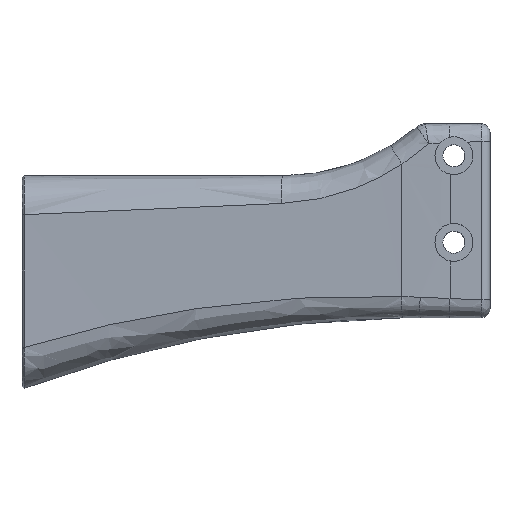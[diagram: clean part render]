
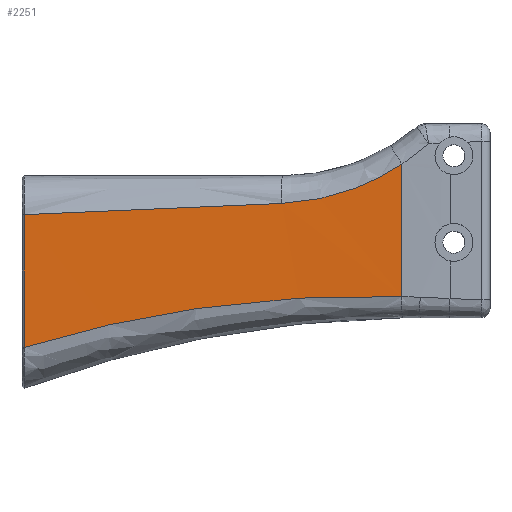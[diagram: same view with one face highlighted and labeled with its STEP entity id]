
A CAD part, left-side view. The second image highlights one B-rep face of the part: STEP entity #2251.
In plain terms, the highlighted cylindrical face has radius 3182.51 mm (diameter 6365.01 mm), a partial arc.
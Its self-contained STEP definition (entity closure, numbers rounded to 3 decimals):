
#116=B_SPLINE_CURVE_WITH_KNOTS('',3,(#3561,#3562,#3563,#3564),
 .UNSPECIFIED.,.F.,.F.,(4,4),(-1.419,-1.417),
 .UNSPECIFIED.);
#125=B_SPLINE_CURVE_WITH_KNOTS('',3,(#3805,#3806,#3807,#3808),
 .UNSPECIFIED.,.F.,.F.,(4,4),(0.05,6.025),
 .UNSPECIFIED.);
#128=B_SPLINE_CURVE_WITH_KNOTS('',3,(#3823,#3824,#3825,#3826,#3827),
 .UNSPECIFIED.,.F.,.F.,(4,1,4),(2.018,7.279,10.884),
 .UNSPECIFIED.);
#129=B_SPLINE_CURVE_WITH_KNOTS('',3,(#3830,#3831,#3832,#3833,#3834),
 .UNSPECIFIED.,.F.,.F.,(4,1,4),(6.025,7.294,8.985),
 .UNSPECIFIED.);
#303=FACE_OUTER_BOUND('',#443,.T.);
#443=EDGE_LOOP('',(#1794,#1795,#1796,#1797,#1798,#1799));
#614=LINE('',#3489,#779);
#631=LINE('',#3829,#796);
#779=VECTOR('',#2795,10.);
#796=VECTOR('',#2820,10.);
#1044=VERTEX_POINT('',#3486);
#1045=VERTEX_POINT('',#3488);
#1047=VERTEX_POINT('',#3537);
#1058=VERTEX_POINT('',#3804);
#1060=VERTEX_POINT('',#3822);
#1061=VERTEX_POINT('',#3828);
#1301=EDGE_CURVE('',#1044,#1045,#614,.T.);
#1307=EDGE_CURVE('',#1045,#1047,#116,.T.);
#1329=EDGE_CURVE('',#1047,#1058,#125,.T.);
#1332=EDGE_CURVE('',#1060,#1044,#128,.T.);
#1333=EDGE_CURVE('',#1061,#1060,#631,.T.);
#1334=EDGE_CURVE('',#1058,#1061,#129,.T.);
#1794=ORIENTED_EDGE('',*,*,#1307,.F.);
#1795=ORIENTED_EDGE('',*,*,#1301,.F.);
#1796=ORIENTED_EDGE('',*,*,#1332,.F.);
#1797=ORIENTED_EDGE('',*,*,#1333,.F.);
#1798=ORIENTED_EDGE('',*,*,#1334,.F.);
#1799=ORIENTED_EDGE('',*,*,#1329,.F.);
#2183=CYLINDRICAL_SURFACE('',#2440,3182.507);
#2251=ADVANCED_FACE('',(#303),#2183,.F.);
#2440=AXIS2_PLACEMENT_3D('',#3821,#2818,#2819);
#2795=DIRECTION('',(0.,0.,1.));
#2818=DIRECTION('center_axis',(0.,0.,-1.));
#2819=DIRECTION('ref_axis',(0.999,-0.041,0.));
#2820=DIRECTION('',(0.,0.,-1.));
#3486=CARTESIAN_POINT('',(0.947,299.5,-160.196));
#3488=CARTESIAN_POINT('',(0.947,299.5,-129.588));
#3489=CARTESIAN_POINT('',(0.947,299.5,-108.588));
#3537=CARTESIAN_POINT('',(0.947,299.5,-129.567));
#3561=CARTESIAN_POINT('Ctrl Pts',(0.947,299.5,-129.588));
#3562=CARTESIAN_POINT('Ctrl Pts',(0.947,299.5,-129.581));
#3563=CARTESIAN_POINT('Ctrl Pts',(0.947,299.5,-129.574));
#3564=CARTESIAN_POINT('Ctrl Pts',(0.947,299.5,-129.567));
#3804=CARTESIAN_POINT('',(-0.33,240.019,-126.981));
#3805=CARTESIAN_POINT('Ctrl Pts',(0.947,299.5,-129.567));
#3806=CARTESIAN_POINT('Ctrl Pts',(0.707,279.673,-128.705));
#3807=CARTESIAN_POINT('Ctrl Pts',(0.282,259.853,-127.843));
#3808=CARTESIAN_POINT('Ctrl Pts',(-0.33,240.019,-126.981));
#3821=CARTESIAN_POINT('Origin',(-3181.326,338.055,-108.588));
#3822=CARTESIAN_POINT('',(-1.304,212.319,-148.474));
#3823=CARTESIAN_POINT('Ctrl Pts',(-1.304,212.319,-148.474));
#3824=CARTESIAN_POINT('Ctrl Pts',(-0.613,229.788,-147.963));
#3825=CARTESIAN_POINT('Ctrl Pts',(0.308,259.316,-149.965));
#3826=CARTESIAN_POINT('Ctrl Pts',(0.808,288.042,-156.7));
#3827=CARTESIAN_POINT('Ctrl Pts',(0.947,299.5,-160.196));
#3828=CARTESIAN_POINT('',(-1.304,212.319,-117.936));
#3829=CARTESIAN_POINT('',(-1.304,212.319,-108.588));
#3830=CARTESIAN_POINT('Ctrl Pts',(-0.33,240.019,-126.981));
#3831=CARTESIAN_POINT('Ctrl Pts',(-0.459,235.809,-126.798));
#3832=CARTESIAN_POINT('Ctrl Pts',(-0.78,226.036,-125.23));
#3833=CARTESIAN_POINT('Ctrl Pts',(-1.119,216.992,-121.063));
#3834=CARTESIAN_POINT('Ctrl Pts',(-1.304,212.319,-117.936));
